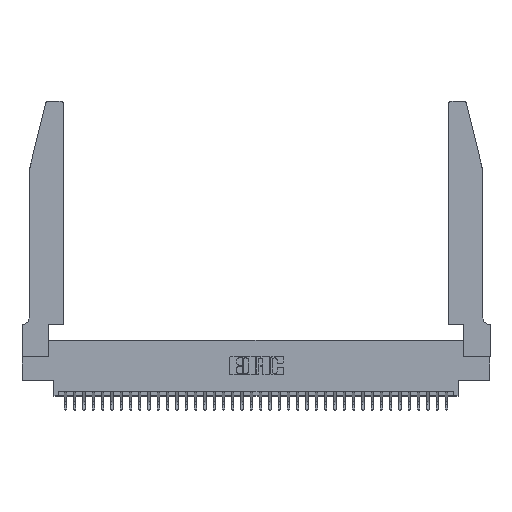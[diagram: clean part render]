
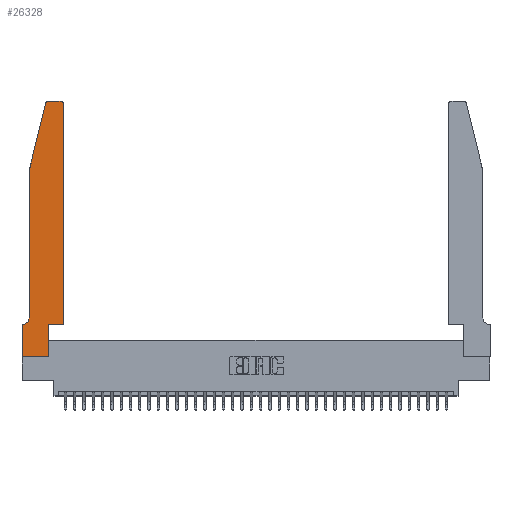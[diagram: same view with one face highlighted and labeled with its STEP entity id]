
A CAD part, top view. The second image highlights one B-rep face of the part: STEP entity #26328.
In plain terms, the highlighted planar face has unit normal (0, 0, 1).
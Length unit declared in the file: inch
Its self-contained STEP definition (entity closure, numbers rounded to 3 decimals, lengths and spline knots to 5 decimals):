
#126 = VERTEX_POINT ( 'NONE', #24120 ) ;
#252 = VECTOR ( 'NONE', #7593, 39.37008 ) ;
#887 = CARTESIAN_POINT ( 'NONE',  ( 0., 0.35, 0.37 ) ) ;
#1696 = VERTEX_POINT ( 'NONE', #11495 ) ;
#3106 = CIRCLE ( 'NONE', #36287, 0.03 ) ;
#3668 = LINE ( 'NONE', #13535, #35027 ) ;
#3840 = CARTESIAN_POINT ( 'NONE',  ( 0.25487, 2.72718, 0.37 ) ) ;
#3994 = ORIENTED_EDGE ( 'NONE', *, *, #33353, .T. ) ;
#4574 = VERTEX_POINT ( 'NONE', #6774 ) ;
#4768 = DIRECTION ( 'NONE',  ( 1., 0., 0. ) ) ;
#4908 = CARTESIAN_POINT ( 'NONE',  ( 0.4505, 0.35, 0.37 ) ) ;
#5073 = CIRCLE ( 'NONE', #20677, 0.03 ) ;
#5261 = CARTESIAN_POINT ( 'NONE',  ( 0.4205, 2.72, 0.37 ) ) ;
#5528 = VERTEX_POINT ( 'NONE', #17958 ) ;
#5864 = EDGE_CURVE ( 'NONE', #5528, #1696, #21879, .T. ) ;
#6175 = VERTEX_POINT ( 'NONE', #32193 ) ;
#6733 = ORIENTED_EDGE ( 'NONE', *, *, #5864, .T. ) ;
#6774 = CARTESIAN_POINT ( 'NONE',  ( 0.284, 2.75, 0.37 ) ) ;
#7593 = DIRECTION ( 'NONE',  ( 1., 0., 0. ) ) ;
#7595 = DIRECTION ( 'NONE',  ( 0., -1., 0. ) ) ;
#7914 = DIRECTION ( 'NONE',  ( 0., 0., 1. ) ) ;
#8053 = VERTEX_POINT ( 'NONE', #9132 ) ;
#8266 = LINE ( 'NONE', #10069, #18298 ) ;
#8601 = DIRECTION ( 'NONE',  ( -1., 0., 0. ) ) ;
#8788 = CIRCLE ( 'NONE', #33242, 0.07 ) ;
#8794 = EDGE_CURVE ( 'NONE', #14705, #4574, #3668, .T. ) ;
#8866 = ORIENTED_EDGE ( 'NONE', *, *, #17423, .T. ) ;
#9132 = CARTESIAN_POINT ( 'NONE',  ( 0.4505, 2.72, 0.37 ) ) ;
#9682 = CARTESIAN_POINT ( 'NONE',  ( 0.4205, 2.75, 0.37 ) ) ;
#10069 = CARTESIAN_POINT ( 'NONE',  ( 0.0755, 2., 0.37 ) ) ;
#10633 = CARTESIAN_POINT ( 'NONE',  ( 0.4505, 0.35, 0.37 ) ) ;
#11495 = CARTESIAN_POINT ( 'NONE',  ( 0.2865, 0., 0.37 ) ) ;
#11807 = ORIENTED_EDGE ( 'NONE', *, *, #32525, .T. ) ;
#12172 = ORIENTED_EDGE ( 'NONE', *, *, #20539, .T. ) ;
#12385 = LINE ( 'NONE', #4908, #21553 ) ;
#12474 = ORIENTED_EDGE ( 'NONE', *, *, #25923, .T. ) ;
#13329 = LINE ( 'NONE', #23750, #30828 ) ;
#13465 = LINE ( 'NONE', #10633, #23615 ) ;
#13535 = CARTESIAN_POINT ( 'NONE',  ( 0.2605, 2.75, 0.37 ) ) ;
#13585 = DIRECTION ( 'NONE',  ( 0., 1., 0. ) ) ;
#14109 = DIRECTION ( 'NONE',  ( 1., 0., 0. ) ) ;
#14705 = VERTEX_POINT ( 'NONE', #9682 ) ;
#15261 = DIRECTION ( 'NONE',  ( 0., 1., 0. ) ) ;
#15271 = EDGE_LOOP ( 'NONE', ( #31535, #18020, #26197, #3994, #22247, #25589, #8866, #6733, #11807, #12172, #12474, #20276 ) ) ;
#15387 = VERTEX_POINT ( 'NONE', #887 ) ;
#15617 = CARTESIAN_POINT ( 'NONE',  ( 0.0755, 2., 0.37 ) ) ;
#15888 = CARTESIAN_POINT ( 'NONE',  ( 0., 0., 0.37 ) ) ;
#17423 = EDGE_CURVE ( 'NONE', #15387, #5528, #37438, .T. ) ;
#17600 = CARTESIAN_POINT ( 'NONE',  ( 0.0055, 0.35, 0.37 ) ) ;
#17929 = DIRECTION ( 'NONE',  ( 1., 0., 0. ) ) ;
#17958 = CARTESIAN_POINT ( 'NONE',  ( 0., 0., 0.37 ) ) ;
#18020 = ORIENTED_EDGE ( 'NONE', *, *, #25341, .T. ) ;
#18087 = AXIS2_PLACEMENT_3D ( 'NONE', #31024, #7914, #31533 ) ;
#18298 = VECTOR ( 'NONE', #21767, 39.37008 ) ;
#19302 = EDGE_CURVE ( 'NONE', #31258, #15387, #35948, .T. ) ;
#19672 = EDGE_CURVE ( 'NONE', #35329, #25235, #13329, .T. ) ;
#20164 = EDGE_CURVE ( 'NONE', #126, #31258, #8788, .T. ) ;
#20276 = ORIENTED_EDGE ( 'NONE', *, *, #32912, .T. ) ;
#20539 = EDGE_CURVE ( 'NONE', #36251, #6175, #12385, .T. ) ;
#20677 = AXIS2_PLACEMENT_3D ( 'NONE', #5261, #25849, #14109 ) ;
#21553 = VECTOR ( 'NONE', #4768, 39.37008 ) ;
#21767 = DIRECTION ( 'NONE',  ( 0., -1., 0. ) ) ;
#21879 = LINE ( 'NONE', #15888, #252 ) ;
#22247 = ORIENTED_EDGE ( 'NONE', *, *, #20164, .T. ) ;
#22708 = CARTESIAN_POINT ( 'NONE',  ( 0.2865, 0.35, 0.37 ) ) ;
#23051 = CARTESIAN_POINT ( 'NONE',  ( 0.0755, 0.35, 0.37 ) ) ;
#23615 = VECTOR ( 'NONE', #13585, 39.37008 ) ;
#23750 = CARTESIAN_POINT ( 'NONE',  ( 0.0755, 2., 0.37 ) ) ;
#24120 = CARTESIAN_POINT ( 'NONE',  ( 0.0755, 0.42, 0.37 ) ) ;
#24547 = FACE_OUTER_BOUND ( 'NONE', #15271, .T. ) ;
#25235 = VERTEX_POINT ( 'NONE', #15617 ) ;
#25341 = EDGE_CURVE ( 'NONE', #4574, #35329, #3106, .T. ) ;
#25589 = ORIENTED_EDGE ( 'NONE', *, *, #19302, .T. ) ;
#25849 = DIRECTION ( 'NONE',  ( 0., 0., 1. ) ) ;
#25923 = EDGE_CURVE ( 'NONE', #6175, #8053, #13465, .T. ) ;
#25936 = VECTOR ( 'NONE', #7595, 39.37008 ) ;
#26197 = ORIENTED_EDGE ( 'NONE', *, *, #19672, .T. ) ;
#26328 = ADVANCED_FACE ( 'NONE', ( #24547 ), #27955, .T. ) ;
#26704 = DIRECTION ( 'NONE',  ( -0.239, -0.971, 0. ) ) ;
#27955 = PLANE ( 'NONE',  #18087 ) ;
#28312 = CARTESIAN_POINT ( 'NONE',  ( 0., 0., 0.37 ) ) ;
#29416 = LINE ( 'NONE', #29944, #32594 ) ;
#29944 = CARTESIAN_POINT ( 'NONE',  ( 0.2865, 0.35, 0.37 ) ) ;
#30136 = CARTESIAN_POINT ( 'NONE',  ( 0.284, 2.72, 0.37 ) ) ;
#30253 = DIRECTION ( 'NONE',  ( 0., 0., 1. ) ) ;
#30828 = VECTOR ( 'NONE', #26704, 39.37008 ) ;
#31024 = CARTESIAN_POINT ( 'NONE',  ( 0., 0.35, 0.37 ) ) ;
#31258 = VERTEX_POINT ( 'NONE', #17600 ) ;
#31533 = DIRECTION ( 'NONE',  ( 1., 0., 0. ) ) ;
#31535 = ORIENTED_EDGE ( 'NONE', *, *, #8794, .T. ) ;
#31744 = DIRECTION ( 'NONE',  ( 0., 0., -1. ) ) ;
#32193 = CARTESIAN_POINT ( 'NONE',  ( 0.4505, 0.35, 0.37 ) ) ;
#32525 = EDGE_CURVE ( 'NONE', #1696, #36251, #29416, .T. ) ;
#32594 = VECTOR ( 'NONE', #15261, 39.37008 ) ;
#32912 = EDGE_CURVE ( 'NONE', #8053, #14705, #5073, .T. ) ;
#33242 = AXIS2_PLACEMENT_3D ( 'NONE', #34441, #31744, #37835 ) ;
#33353 = EDGE_CURVE ( 'NONE', #25235, #126, #8266, .T. ) ;
#34251 = DIRECTION ( 'NONE',  ( -1., 0., 0. ) ) ;
#34441 = CARTESIAN_POINT ( 'NONE',  ( 0.0055, 0.42, 0.37 ) ) ;
#35027 = VECTOR ( 'NONE', #8601, 39.37008 ) ;
#35329 = VERTEX_POINT ( 'NONE', #3840 ) ;
#35948 = LINE ( 'NONE', #23051, #37833 ) ;
#36251 = VERTEX_POINT ( 'NONE', #22708 ) ;
#36287 = AXIS2_PLACEMENT_3D ( 'NONE', #30136, #30253, #17929 ) ;
#37438 = LINE ( 'NONE', #28312, #25936 ) ;
#37833 = VECTOR ( 'NONE', #34251, 39.37008 ) ;
#37835 = DIRECTION ( 'NONE',  ( -1., 0., 0. ) ) ;
